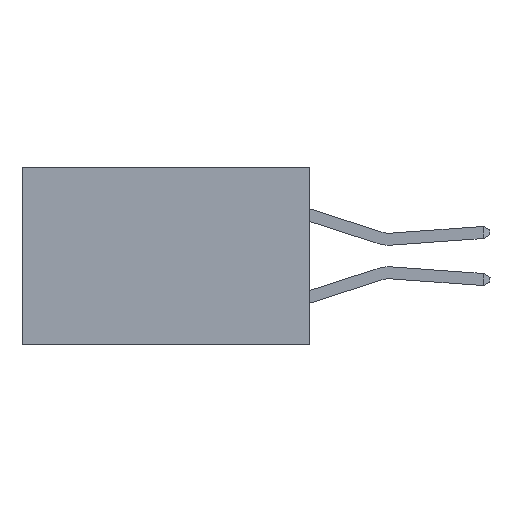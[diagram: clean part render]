
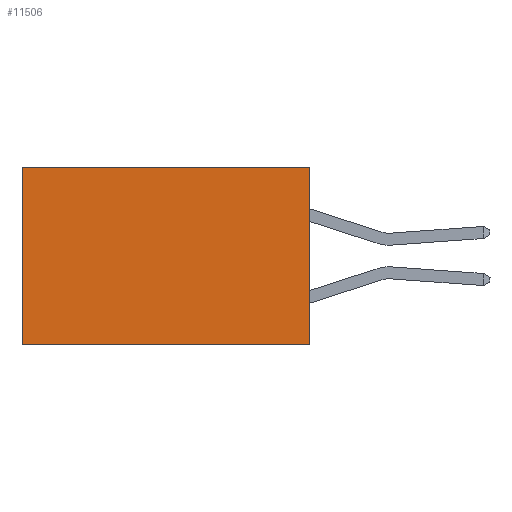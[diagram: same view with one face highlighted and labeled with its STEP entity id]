
A CAD part, left-side view. The second image highlights one B-rep face of the part: STEP entity #11506.
In plain terms, the highlighted planar face has unit normal (-1, 0, 0).
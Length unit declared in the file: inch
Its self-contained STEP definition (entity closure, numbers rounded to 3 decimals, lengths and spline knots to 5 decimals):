
#44 = CARTESIAN_POINT ( 'NONE',  ( 0.298, 0.6, 0. ) ) ;
#121 = LINE ( 'NONE', #6916, #7196 ) ;
#235 = DIRECTION ( 'NONE',  ( 0., 0., -1. ) ) ;
#303 = VECTOR ( 'NONE', #12055, 39.37008 ) ;
#332 = VERTEX_POINT ( 'NONE', #10806 ) ;
#375 = VERTEX_POINT ( 'NONE', #44 ) ;
#803 = CARTESIAN_POINT ( 'NONE',  ( 0.298, 0., -0.37 ) ) ;
#1713 = CARTESIAN_POINT ( 'NONE',  ( 0.298, 0.6, 0. ) ) ;
#2272 = AXIS2_PLACEMENT_3D ( 'NONE', #9257, #9303, #235 ) ;
#2343 = VERTEX_POINT ( 'NONE', #4109 ) ;
#2591 = EDGE_CURVE ( 'NONE', #2343, #375, #12081, .T. ) ;
#2748 = FACE_OUTER_BOUND ( 'NONE', #8869, .T. ) ;
#3258 = EDGE_CURVE ( 'NONE', #2343, #332, #121, .T. ) ;
#3305 = VERTEX_POINT ( 'NONE', #9583 ) ;
#3637 = DIRECTION ( 'NONE',  ( 0., 0., -1. ) ) ;
#4109 = CARTESIAN_POINT ( 'NONE',  ( 0.298, 0., 0. ) ) ;
#4828 = ORIENTED_EDGE ( 'NONE', *, *, #2591, .T. ) ;
#5262 = PLANE ( 'NONE',  #2272 ) ;
#5511 = VECTOR ( 'NONE', #9569, 39.37008 ) ;
#6111 = DIRECTION ( 'NONE',  ( 0., 0., -1. ) ) ;
#6637 = ORIENTED_EDGE ( 'NONE', *, *, #3258, .F. ) ;
#6913 = CARTESIAN_POINT ( 'NONE',  ( 0.298, 0., 0. ) ) ;
#6916 = CARTESIAN_POINT ( 'NONE',  ( 0.298, 0., 0. ) ) ;
#7196 = VECTOR ( 'NONE', #6111, 39.37008 ) ;
#8304 = EDGE_CURVE ( 'NONE', #375, #3305, #12581, .T. ) ;
#8869 = EDGE_LOOP ( 'NONE', ( #9943, #9322, #6637, #4828 ) ) ;
#9257 = CARTESIAN_POINT ( 'NONE',  ( 0.298, 0., 0. ) ) ;
#9303 = DIRECTION ( 'NONE',  ( 1., 0., 0. ) ) ;
#9322 = ORIENTED_EDGE ( 'NONE', *, *, #12800, .F. ) ;
#9569 = DIRECTION ( 'NONE',  ( 0., 1., 0. ) ) ;
#9583 = CARTESIAN_POINT ( 'NONE',  ( 0.298, 0.6, -0.37 ) ) ;
#9922 = VECTOR ( 'NONE', #3637, 39.37008 ) ;
#9943 = ORIENTED_EDGE ( 'NONE', *, *, #8304, .T. ) ;
#10806 = CARTESIAN_POINT ( 'NONE',  ( 0.298, 0., -0.37 ) ) ;
#11506 = ADVANCED_FACE ( 'NONE', ( #2748 ), #5262, .F. ) ;
#11925 = LINE ( 'NONE', #803, #5511 ) ;
#12055 = DIRECTION ( 'NONE',  ( 0., 1., 0. ) ) ;
#12081 = LINE ( 'NONE', #6913, #303 ) ;
#12581 = LINE ( 'NONE', #1713, #9922 ) ;
#12800 = EDGE_CURVE ( 'NONE', #332, #3305, #11925, .T. ) ;
